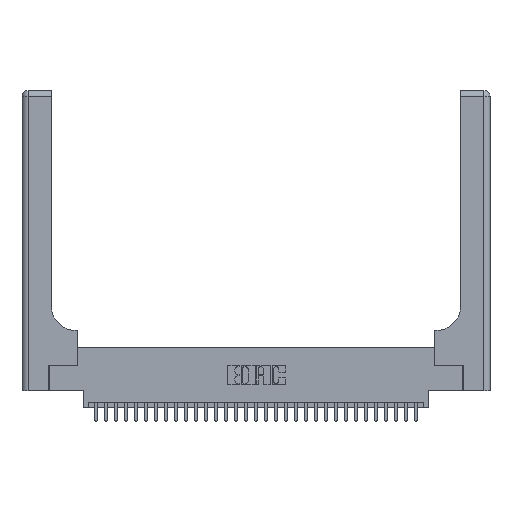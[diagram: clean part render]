
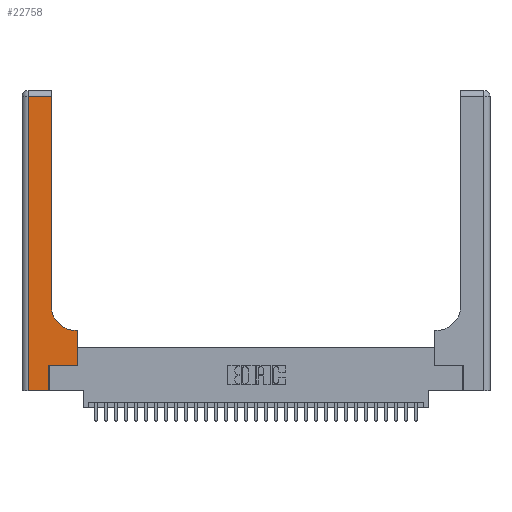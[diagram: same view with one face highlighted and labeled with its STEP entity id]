
A CAD part, top view. The second image highlights one B-rep face of the part: STEP entity #22758.
In plain terms, the highlighted planar face has unit normal (0, 0, 1).
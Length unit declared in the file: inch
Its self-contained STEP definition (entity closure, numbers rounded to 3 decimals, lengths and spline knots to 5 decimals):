
#896 = CARTESIAN_POINT ( 'NONE',  ( 0.2915, 0.6, 0.37 ) ) ;
#905 = PLANE ( 'NONE',  #4817 ) ;
#1077 = LINE ( 'NONE', #24369, #2646 ) ;
#1208 = DIRECTION ( 'NONE',  ( 1., 0., 0. ) ) ;
#1218 = ORIENTED_EDGE ( 'NONE', *, *, #6983, .T. ) ;
#1688 = CARTESIAN_POINT ( 'NONE',  ( 0.2915, 2.94, 0.37 ) ) ;
#2097 = CARTESIAN_POINT ( 'NONE',  ( 0.269, 0.25, 0.37 ) ) ;
#2646 = VECTOR ( 'NONE', #9440, 39.37008 ) ;
#2676 = EDGE_CURVE ( 'NONE', #24826, #6440, #19384, .T. ) ;
#2929 = LINE ( 'NONE', #896, #26034 ) ;
#3059 = VECTOR ( 'NONE', #4413, 39.37008 ) ;
#3157 = EDGE_CURVE ( 'NONE', #21653, #18632, #26340, .T. ) ;
#3220 = CIRCLE ( 'NONE', #24274, 0.25 ) ;
#3761 = DIRECTION ( 'NONE',  ( 0., 0., -1. ) ) ;
#3843 = LINE ( 'NONE', #2097, #3059 ) ;
#4413 = DIRECTION ( 'NONE',  ( 1., 0., 0. ) ) ;
#4790 = CARTESIAN_POINT ( 'NONE',  ( 0.06, 2.94, 0.37 ) ) ;
#4817 = AXIS2_PLACEMENT_3D ( 'NONE', #19214, #3761, #28836 ) ;
#5380 = FACE_OUTER_BOUND ( 'NONE', #30561, .T. ) ;
#5636 = VECTOR ( 'NONE', #13249, 39.37008 ) ;
#5674 = ORIENTED_EDGE ( 'NONE', *, *, #2676, .T. ) ;
#6440 = VERTEX_POINT ( 'NONE', #1688 ) ;
#6983 = EDGE_CURVE ( 'NONE', #11724, #27902, #27212, .T. ) ;
#7199 = CARTESIAN_POINT ( 'NONE',  ( 0.5585, 0.25, 0.37 ) ) ;
#7359 = VERTEX_POINT ( 'NONE', #25663 ) ;
#8536 = EDGE_CURVE ( 'NONE', #31459, #24826, #3220, .T. ) ;
#9440 = DIRECTION ( 'NONE',  ( 0., -1., 0. ) ) ;
#9606 = CARTESIAN_POINT ( 'NONE',  ( 0.5585, 0.6, 0.37 ) ) ;
#9920 = ORIENTED_EDGE ( 'NONE', *, *, #13473, .T. ) ;
#10841 = CARTESIAN_POINT ( 'NONE',  ( 0.5415, 0.6, 0.37 ) ) ;
#10862 = ORIENTED_EDGE ( 'NONE', *, *, #28935, .T. ) ;
#10904 = DIRECTION ( 'NONE',  ( 0., 0., -1. ) ) ;
#11313 = CARTESIAN_POINT ( 'NONE',  ( 0.2915, 3., 0.37 ) ) ;
#11724 = VERTEX_POINT ( 'NONE', #12324 ) ;
#12146 = CARTESIAN_POINT ( 'NONE',  ( 0., 2.94, 0.37 ) ) ;
#12324 = CARTESIAN_POINT ( 'NONE',  ( 0.06, 0., 0.37 ) ) ;
#12395 = VECTOR ( 'NONE', #27387, 39.37008 ) ;
#13249 = DIRECTION ( 'NONE',  ( 0., 1., 0. ) ) ;
#13352 = CARTESIAN_POINT ( 'NONE',  ( 0.269, 0., 0.37 ) ) ;
#13473 = EDGE_CURVE ( 'NONE', #17886, #11724, #1077, .T. ) ;
#13994 = ORIENTED_EDGE ( 'NONE', *, *, #8536, .T. ) ;
#16227 = LINE ( 'NONE', #13352, #5636 ) ;
#16965 = EDGE_CURVE ( 'NONE', #27902, #7359, #16227, .T. ) ;
#17886 = VERTEX_POINT ( 'NONE', #4790 ) ;
#18262 = ORIENTED_EDGE ( 'NONE', *, *, #27215, .T. ) ;
#18632 = VERTEX_POINT ( 'NONE', #9606 ) ;
#18665 = VECTOR ( 'NONE', #26567, 39.37008 ) ;
#19214 = CARTESIAN_POINT ( 'NONE',  ( 0., 3., 0.37 ) ) ;
#19384 = LINE ( 'NONE', #11313, #21727 ) ;
#19799 = LINE ( 'NONE', #12146, #12395 ) ;
#20441 = ORIENTED_EDGE ( 'NONE', *, *, #31872, .T. ) ;
#21653 = VERTEX_POINT ( 'NONE', #26588 ) ;
#21727 = VECTOR ( 'NONE', #31754, 39.37008 ) ;
#22055 = VECTOR ( 'NONE', #26874, 39.37008 ) ;
#22758 = ADVANCED_FACE ( 'NONE', ( #5380 ), #905, .F. ) ;
#23333 = CARTESIAN_POINT ( 'NONE',  ( 0.5415, 0.85, 0.37 ) ) ;
#24274 = AXIS2_PLACEMENT_3D ( 'NONE', #23333, #10904, #1208 ) ;
#24369 = CARTESIAN_POINT ( 'NONE',  ( 0.06, 3., 0.37 ) ) ;
#24826 = VERTEX_POINT ( 'NONE', #27553 ) ;
#25663 = CARTESIAN_POINT ( 'NONE',  ( 0.269, 0.25, 0.37 ) ) ;
#26034 = VECTOR ( 'NONE', #28517, 39.37008 ) ;
#26340 = LINE ( 'NONE', #7199, #22055 ) ;
#26567 = DIRECTION ( 'NONE',  ( 1., 0., 0. ) ) ;
#26588 = CARTESIAN_POINT ( 'NONE',  ( 0.5585, 0.25, 0.37 ) ) ;
#26874 = DIRECTION ( 'NONE',  ( 0., 1., 0. ) ) ;
#27212 = LINE ( 'NONE', #31984, #18665 ) ;
#27215 = EDGE_CURVE ( 'NONE', #7359, #21653, #3843, .T. ) ;
#27338 = CARTESIAN_POINT ( 'NONE',  ( 0.269, 0., 0.37 ) ) ;
#27387 = DIRECTION ( 'NONE',  ( -1., 0., 0. ) ) ;
#27553 = CARTESIAN_POINT ( 'NONE',  ( 0.2915, 0.85, 0.37 ) ) ;
#27902 = VERTEX_POINT ( 'NONE', #27338 ) ;
#28517 = DIRECTION ( 'NONE',  ( -1., 0., 0. ) ) ;
#28836 = DIRECTION ( 'NONE',  ( -1., 0., 0. ) ) ;
#28935 = EDGE_CURVE ( 'NONE', #18632, #31459, #2929, .T. ) ;
#30561 = EDGE_LOOP ( 'NONE', ( #5674, #20441, #9920, #1218, #31627, #18262, #30885, #10862, #13994 ) ) ;
#30885 = ORIENTED_EDGE ( 'NONE', *, *, #3157, .T. ) ;
#31459 = VERTEX_POINT ( 'NONE', #10841 ) ;
#31627 = ORIENTED_EDGE ( 'NONE', *, *, #16965, .T. ) ;
#31754 = DIRECTION ( 'NONE',  ( 0., 1., 0. ) ) ;
#31872 = EDGE_CURVE ( 'NONE', #6440, #17886, #19799, .T. ) ;
#31984 = CARTESIAN_POINT ( 'NONE',  ( 0., 0., 0.37 ) ) ;
